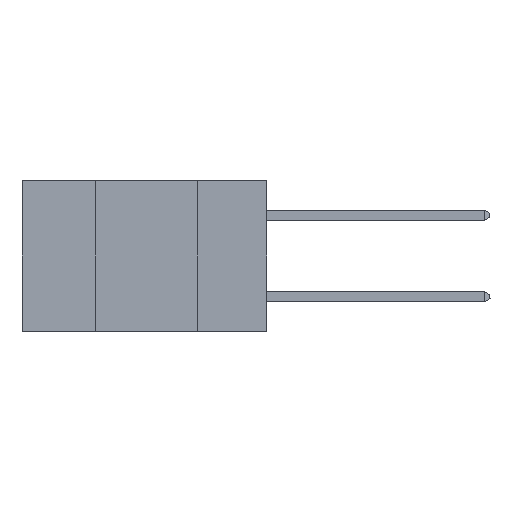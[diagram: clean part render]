
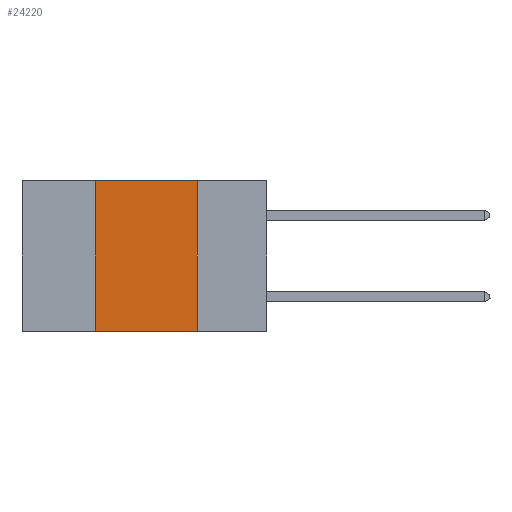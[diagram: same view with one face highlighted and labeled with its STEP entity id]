
A CAD part, left-side view. The second image highlights one B-rep face of the part: STEP entity #24220.
In plain terms, the highlighted planar face has unit normal (-1, 0, 0).
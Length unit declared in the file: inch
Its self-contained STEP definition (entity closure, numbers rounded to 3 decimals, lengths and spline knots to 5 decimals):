
#517 = EDGE_CURVE ( 'NONE', #17661, #19896, #12333, .T. ) ;
#1656 = VECTOR ( 'NONE', #19231, 39.37008 ) ;
#2470 = VERTEX_POINT ( 'NONE', #14763 ) ;
#2864 = CARTESIAN_POINT ( 'NONE',  ( 0., 0.6, -0.37 ) ) ;
#3185 = CARTESIAN_POINT ( 'NONE',  ( 0., 0.6, 0. ) ) ;
#4554 = CARTESIAN_POINT ( 'NONE',  ( 0., 0.17, 0. ) ) ;
#5255 = LINE ( 'NONE', #7857, #25579 ) ;
#6969 = LINE ( 'NONE', #4554, #25367 ) ;
#7767 = DIRECTION ( 'NONE',  ( 0., 0., 1. ) ) ;
#7857 = CARTESIAN_POINT ( 'NONE',  ( 0., 0.42, 0. ) ) ;
#9425 = DIRECTION ( 'NONE',  ( 0., 0., -1. ) ) ;
#9448 = VECTOR ( 'NONE', #10803, 39.37008 ) ;
#10803 = DIRECTION ( 'NONE',  ( 0., -1., 0. ) ) ;
#10889 = FACE_OUTER_BOUND ( 'NONE', #23811, .T. ) ;
#10921 = CARTESIAN_POINT ( 'NONE',  ( 0., 0.42, -0.37 ) ) ;
#10962 = AXIS2_PLACEMENT_3D ( 'NONE', #3185, #17866, #9425 ) ;
#12333 = LINE ( 'NONE', #2864, #9448 ) ;
#12756 = ORIENTED_EDGE ( 'NONE', *, *, #26052, .F. ) ;
#13353 = ORIENTED_EDGE ( 'NONE', *, *, #21702, .F. ) ;
#13921 = ORIENTED_EDGE ( 'NONE', *, *, #23969, .F. ) ;
#14533 = VERTEX_POINT ( 'NONE', #22385 ) ;
#14763 = CARTESIAN_POINT ( 'NONE',  ( 0., 0.42, 0. ) ) ;
#14864 = LINE ( 'NONE', #19316, #1656 ) ;
#17661 = VERTEX_POINT ( 'NONE', #10921 ) ;
#17866 = DIRECTION ( 'NONE',  ( 1., 0., 0. ) ) ;
#18726 = DIRECTION ( 'NONE',  ( 0., 0., -1. ) ) ;
#19231 = DIRECTION ( 'NONE',  ( 0., -1., 0. ) ) ;
#19316 = CARTESIAN_POINT ( 'NONE',  ( 0., 0.6, 0. ) ) ;
#19338 = ORIENTED_EDGE ( 'NONE', *, *, #517, .T. ) ;
#19896 = VERTEX_POINT ( 'NONE', #20180 ) ;
#20180 = CARTESIAN_POINT ( 'NONE',  ( 0., 0.17, -0.37 ) ) ;
#21702 = EDGE_CURVE ( 'NONE', #2470, #14533, #14864, .T. ) ;
#22385 = CARTESIAN_POINT ( 'NONE',  ( 0., 0.17, 0. ) ) ;
#23811 = EDGE_LOOP ( 'NONE', ( #13921, #13353, #12756, #19338 ) ) ;
#23969 = EDGE_CURVE ( 'NONE', #14533, #19896, #6969, .T. ) ;
#24220 = ADVANCED_FACE ( 'NONE', ( #10889 ), #26138, .F. ) ;
#25367 = VECTOR ( 'NONE', #18726, 39.37008 ) ;
#25579 = VECTOR ( 'NONE', #7767, 39.37008 ) ;
#26052 = EDGE_CURVE ( 'NONE', #17661, #2470, #5255, .T. ) ;
#26138 = PLANE ( 'NONE',  #10962 ) ;
